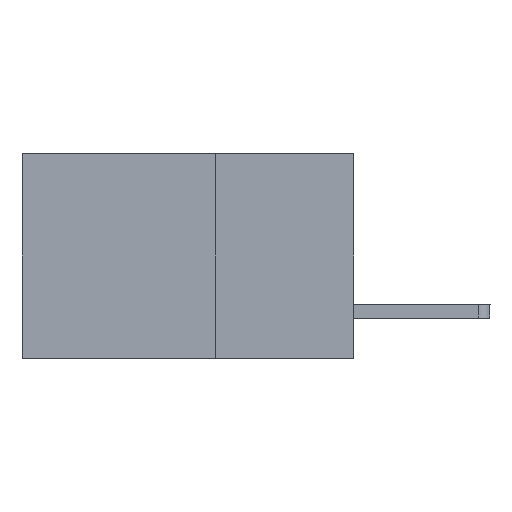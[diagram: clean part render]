
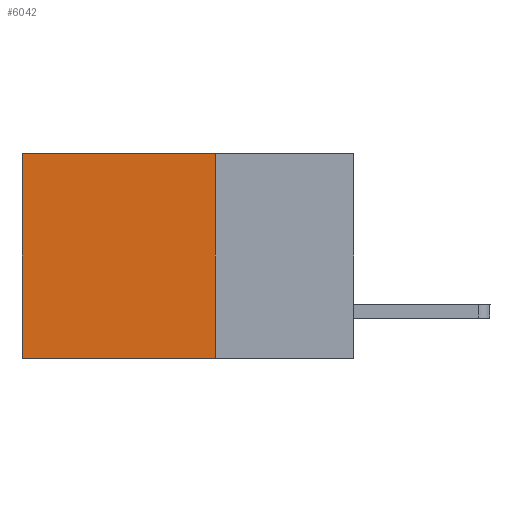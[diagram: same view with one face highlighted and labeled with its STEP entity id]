
A CAD part, left-side view. The second image highlights one B-rep face of the part: STEP entity #6042.
In plain terms, the highlighted planar face has unit normal (-1, 0, 0).
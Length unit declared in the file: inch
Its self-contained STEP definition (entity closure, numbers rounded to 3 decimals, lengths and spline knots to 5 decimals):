
#20 = CARTESIAN_POINT ( 'NONE',  ( 0.2875, 0.6, 0. ) ) ;
#44 = VERTEX_POINT ( 'NONE', #110 ) ;
#110 = CARTESIAN_POINT ( 'NONE',  ( 0.2875, 0.6, -0.37 ) ) ;
#700 = VECTOR ( 'NONE', #4421, 39.37008 ) ;
#1421 = CARTESIAN_POINT ( 'NONE',  ( 0.2875, 0.25, 0. ) ) ;
#2003 = VECTOR ( 'NONE', #5553, 39.37008 ) ;
#2078 = FACE_OUTER_BOUND ( 'NONE', #5158, .T. ) ;
#2112 = CARTESIAN_POINT ( 'NONE',  ( 0.2875, 0.25, -0.37 ) ) ;
#2551 = DIRECTION ( 'NONE',  ( 1., 0., 0. ) ) ;
#2584 = LINE ( 'NONE', #3501, #700 ) ;
#2635 = LINE ( 'NONE', #3132, #9508 ) ;
#3132 = CARTESIAN_POINT ( 'NONE',  ( 0.2875, 0.25, 0. ) ) ;
#3133 = LINE ( 'NONE', #6542, #4771 ) ;
#3211 = VERTEX_POINT ( 'NONE', #10371 ) ;
#3321 = ORIENTED_EDGE ( 'NONE', *, *, #10763, .F. ) ;
#3344 = DIRECTION ( 'NONE',  ( 0., 0., -1. ) ) ;
#3501 = CARTESIAN_POINT ( 'NONE',  ( 0.2875, 0.25, 0. ) ) ;
#3731 = DIRECTION ( 'NONE',  ( 0., 0., -1. ) ) ;
#4154 = ORIENTED_EDGE ( 'NONE', *, *, #8795, .F. ) ;
#4227 = PLANE ( 'NONE',  #7811 ) ;
#4421 = DIRECTION ( 'NONE',  ( 0., 1., 0. ) ) ;
#4770 = VERTEX_POINT ( 'NONE', #20 ) ;
#4771 = VECTOR ( 'NONE', #4841, 39.37008 ) ;
#4841 = DIRECTION ( 'NONE',  ( 0., 0., -1. ) ) ;
#4851 = LINE ( 'NONE', #2112, #2003 ) ;
#5158 = EDGE_LOOP ( 'NONE', ( #9822, #4154, #3321, #10844 ) ) ;
#5424 = EDGE_CURVE ( 'NONE', #4770, #44, #3133, .T. ) ;
#5553 = DIRECTION ( 'NONE',  ( 0., 1., 0. ) ) ;
#5564 = EDGE_CURVE ( 'NONE', #8506, #4770, #2584, .T. ) ;
#6042 = ADVANCED_FACE ( 'NONE', ( #2078 ), #4227, .F. ) ;
#6542 = CARTESIAN_POINT ( 'NONE',  ( 0.2875, 0.6, 0. ) ) ;
#7811 = AXIS2_PLACEMENT_3D ( 'NONE', #8496, #2551, #3344 ) ;
#8496 = CARTESIAN_POINT ( 'NONE',  ( 0.2875, 0.25, 0. ) ) ;
#8506 = VERTEX_POINT ( 'NONE', #1421 ) ;
#8795 = EDGE_CURVE ( 'NONE', #3211, #44, #4851, .T. ) ;
#9508 = VECTOR ( 'NONE', #3731, 39.37008 ) ;
#9822 = ORIENTED_EDGE ( 'NONE', *, *, #5424, .T. ) ;
#10371 = CARTESIAN_POINT ( 'NONE',  ( 0.2875, 0.25, -0.37 ) ) ;
#10763 = EDGE_CURVE ( 'NONE', #8506, #3211, #2635, .T. ) ;
#10844 = ORIENTED_EDGE ( 'NONE', *, *, #5564, .T. ) ;
